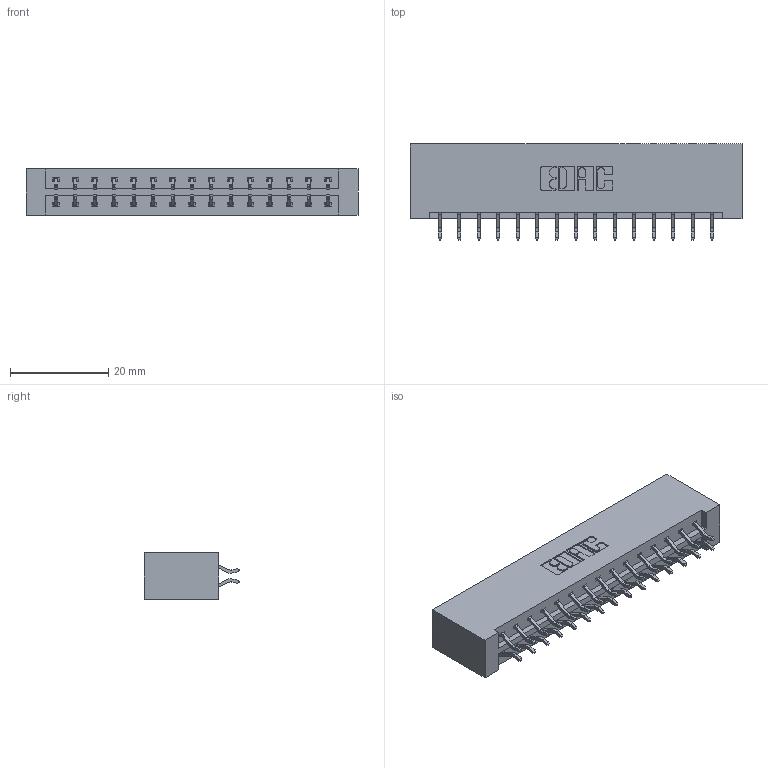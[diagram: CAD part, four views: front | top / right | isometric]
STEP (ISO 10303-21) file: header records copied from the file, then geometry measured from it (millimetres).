
FILE_DESCRIPTION (( 'STEP AP203' ), '1' );
FILE_NAME ('333-030-556-201.STEP', '2018-08-02T18:49:28', ( '' ), ( '' ), 'SwSTEP 2.0', 'SolidWorks 2016', '' );
FILE_SCHEMA (( 'CONFIG_CONTROL_DESIGN' ));
Length unit declared in the file: inch
Products named in the file (3): 333-030-556-201; 333 Part_Lugless; 345-292-001_556 Tail
Assembly tree (31 placements, depth 2):
  333-030-556-201
    333 Part_Lugless
    345-292-001_556 Tail  x30
Bounding box: 67.69 x 19.57 x 9.4 mm (x, y, z)
Volume: 7289.4 mm3; surface area: 8322.5 mm2
Topology: 31 solids, 31 shells, 1846 faces, 5477 edges, 3610 vertices
Faces by surface type: plane 1266, cylinder 580
Entity records: 13085 total; most frequent: CARTESIAN_POINT 2214, ORIENTED_EDGE 2138, DIRECTION 1921, EDGE_CURVE 1069, LINE 941, VECTOR 941, VERTEX_POINT 710, AXIS2_PLACEMENT_3D 490
